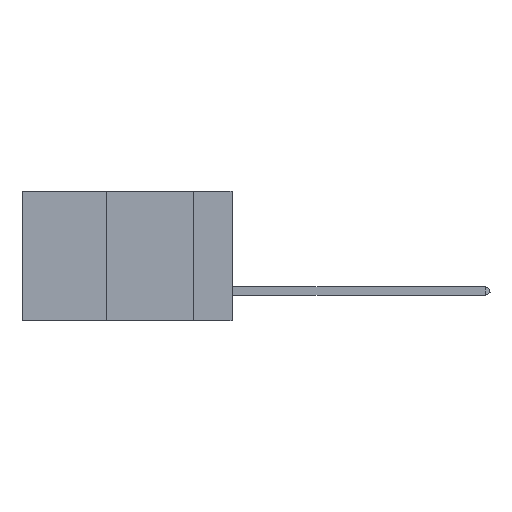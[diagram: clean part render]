
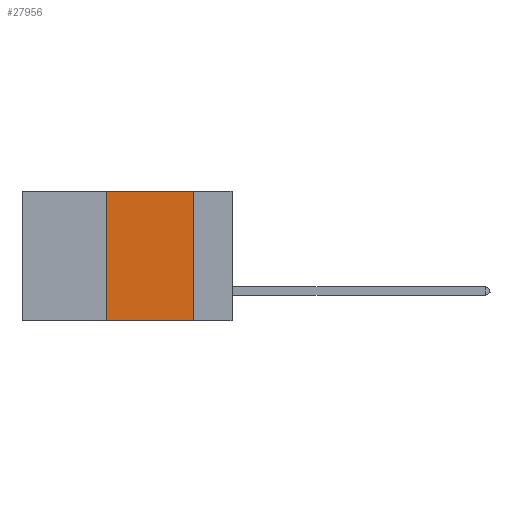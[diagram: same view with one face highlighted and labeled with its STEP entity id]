
A CAD part, left-side view. The second image highlights one B-rep face of the part: STEP entity #27956.
In plain terms, the highlighted planar face has unit normal (-1, 0, 0).
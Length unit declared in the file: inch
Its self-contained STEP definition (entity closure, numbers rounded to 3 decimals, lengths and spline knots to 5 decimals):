
#294 = EDGE_CURVE ( 'NONE', #29011, #14931, #19322, .T. ) ;
#1486 = VECTOR ( 'NONE', #33244, 39.37008 ) ;
#1488 = ORIENTED_EDGE ( 'NONE', *, *, #294, .T. ) ;
#1807 = ORIENTED_EDGE ( 'NONE', *, *, #30780, .F. ) ;
#3127 = VERTEX_POINT ( 'NONE', #7924 ) ;
#3472 = ORIENTED_EDGE ( 'NONE', *, *, #36113, .F. ) ;
#4886 = ORIENTED_EDGE ( 'NONE', *, *, #25260, .F. ) ;
#7924 = CARTESIAN_POINT ( 'NONE',  ( 0., 0.11, 0. ) ) ;
#8829 = AXIS2_PLACEMENT_3D ( 'NONE', #32881, #11918, #35993 ) ;
#9292 = VERTEX_POINT ( 'NONE', #12178 ) ;
#11478 = DIRECTION ( 'NONE',  ( 0., -1., 0. ) ) ;
#11724 = PLANE ( 'NONE',  #8829 ) ;
#11918 = DIRECTION ( 'NONE',  ( 1., 0., 0. ) ) ;
#12178 = CARTESIAN_POINT ( 'NONE',  ( 0., 0.36, 0. ) ) ;
#12653 = LINE ( 'NONE', #24507, #1486 ) ;
#13686 = CARTESIAN_POINT ( 'NONE',  ( 0., 0.6, -0.37 ) ) ;
#14792 = LINE ( 'NONE', #18456, #15080 ) ;
#14931 = VERTEX_POINT ( 'NONE', #24524 ) ;
#15080 = VECTOR ( 'NONE', #20816, 39.37008 ) ;
#18456 = CARTESIAN_POINT ( 'NONE',  ( 0., 0.36, 0. ) ) ;
#19322 = LINE ( 'NONE', #13686, #21262 ) ;
#20816 = DIRECTION ( 'NONE',  ( 0., 0., 1. ) ) ;
#21262 = VECTOR ( 'NONE', #31174, 39.37008 ) ;
#21323 = EDGE_LOOP ( 'NONE', ( #1807, #3472, #4886, #1488 ) ) ;
#21978 = VECTOR ( 'NONE', #11478, 39.37008 ) ;
#23135 = LINE ( 'NONE', #34613, #21978 ) ;
#24507 = CARTESIAN_POINT ( 'NONE',  ( 0., 0.11, 0. ) ) ;
#24524 = CARTESIAN_POINT ( 'NONE',  ( 0., 0.11, -0.37 ) ) ;
#25260 = EDGE_CURVE ( 'NONE', #29011, #9292, #14792, .T. ) ;
#27956 = ADVANCED_FACE ( 'NONE', ( #32128 ), #11724, .F. ) ;
#29011 = VERTEX_POINT ( 'NONE', #30800 ) ;
#30780 = EDGE_CURVE ( 'NONE', #3127, #14931, #12653, .T. ) ;
#30800 = CARTESIAN_POINT ( 'NONE',  ( 0., 0.36, -0.37 ) ) ;
#31174 = DIRECTION ( 'NONE',  ( 0., -1., 0. ) ) ;
#32128 = FACE_OUTER_BOUND ( 'NONE', #21323, .T. ) ;
#32881 = CARTESIAN_POINT ( 'NONE',  ( 0., 0.6, 0. ) ) ;
#33244 = DIRECTION ( 'NONE',  ( 0., 0., -1. ) ) ;
#34613 = CARTESIAN_POINT ( 'NONE',  ( 0., 0.6, 0. ) ) ;
#35993 = DIRECTION ( 'NONE',  ( 0., 0., -1. ) ) ;
#36113 = EDGE_CURVE ( 'NONE', #9292, #3127, #23135, .T. ) ;
